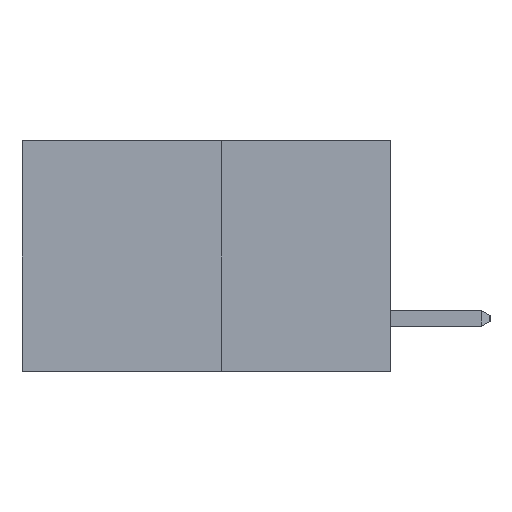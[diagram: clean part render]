
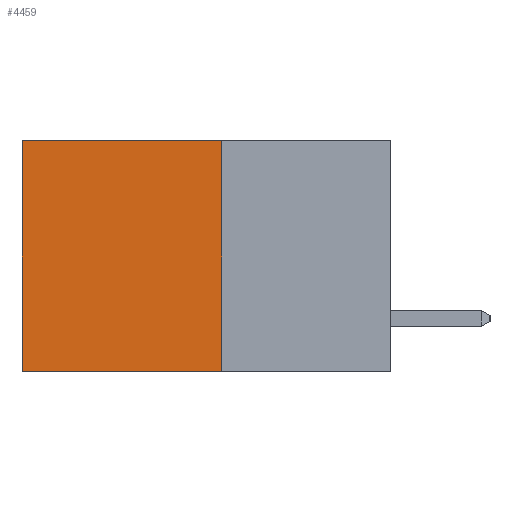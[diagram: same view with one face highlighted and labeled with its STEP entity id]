
A CAD part, left-side view. The second image highlights one B-rep face of the part: STEP entity #4459.
In plain terms, the highlighted planar face has unit normal (-1, 0, 0).
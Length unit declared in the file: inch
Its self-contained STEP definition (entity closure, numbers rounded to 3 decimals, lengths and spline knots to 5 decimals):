
#41 = FACE_OUTER_BOUND ( 'NONE', #4753, .T. ) ;
#660 = VECTOR ( 'NONE', #13528, 39.37008 ) ;
#2257 = CARTESIAN_POINT ( 'NONE',  ( 0.277, 0.27, 0. ) ) ;
#2770 = CARTESIAN_POINT ( 'NONE',  ( 0.277, 0.59, -0.37 ) ) ;
#2908 = CARTESIAN_POINT ( 'NONE',  ( 0.277, 0.27, 0. ) ) ;
#2916 = VERTEX_POINT ( 'NONE', #6749 ) ;
#3190 = LINE ( 'NONE', #10766, #14870 ) ;
#3522 = VERTEX_POINT ( 'NONE', #2257 ) ;
#3648 = EDGE_CURVE ( 'NONE', #2916, #9397, #7498, .T. ) ;
#4135 = DIRECTION ( 'NONE',  ( 0., 1., 0. ) ) ;
#4351 = DIRECTION ( 'NONE',  ( 0., 0., -1. ) ) ;
#4369 = DIRECTION ( 'NONE',  ( 1., 0., 0. ) ) ;
#4402 = CARTESIAN_POINT ( 'NONE',  ( 0.277, 0.27, -0.37 ) ) ;
#4459 = ADVANCED_FACE ( 'NONE', ( #41 ), #4654, .F. ) ;
#4654 = PLANE ( 'NONE',  #10296 ) ;
#4753 = EDGE_LOOP ( 'NONE', ( #5326, #5476, #5497, #5720 ) ) ;
#5326 = ORIENTED_EDGE ( 'NONE', *, *, #3648, .T. ) ;
#5476 = ORIENTED_EDGE ( 'NONE', *, *, #12457, .F. ) ;
#5497 = ORIENTED_EDGE ( 'NONE', *, *, #13616, .F. ) ;
#5720 = ORIENTED_EDGE ( 'NONE', *, *, #10115, .T. ) ;
#5869 = VECTOR ( 'NONE', #4135, 39.37008 ) ;
#6749 = CARTESIAN_POINT ( 'NONE',  ( 0.277, 0.59, 0. ) ) ;
#6946 = VECTOR ( 'NONE', #14303, 39.37008 ) ;
#7498 = LINE ( 'NONE', #13860, #660 ) ;
#8808 = CARTESIAN_POINT ( 'NONE',  ( 0.277, 0.27, -0.37 ) ) ;
#8969 = VERTEX_POINT ( 'NONE', #9063 ) ;
#9063 = CARTESIAN_POINT ( 'NONE',  ( 0.277, 0.27, -0.37 ) ) ;
#9264 = LINE ( 'NONE', #2908, #5869 ) ;
#9397 = VERTEX_POINT ( 'NONE', #2770 ) ;
#10115 = EDGE_CURVE ( 'NONE', #3522, #2916, #9264, .T. ) ;
#10296 = AXIS2_PLACEMENT_3D ( 'NONE', #4402, #4369, #4351 ) ;
#10766 = CARTESIAN_POINT ( 'NONE',  ( 0.277, 0.27, -0.37 ) ) ;
#12457 = EDGE_CURVE ( 'NONE', #8969, #9397, #13299, .T. ) ;
#13299 = LINE ( 'NONE', #8808, #6946 ) ;
#13528 = DIRECTION ( 'NONE',  ( 0., 0., -1. ) ) ;
#13616 = EDGE_CURVE ( 'NONE', #3522, #8969, #3190, .T. ) ;
#13860 = CARTESIAN_POINT ( 'NONE',  ( 0.277, 0.59, -0.37 ) ) ;
#14068 = DIRECTION ( 'NONE',  ( 0., 0., -1. ) ) ;
#14303 = DIRECTION ( 'NONE',  ( 0., 1., 0. ) ) ;
#14870 = VECTOR ( 'NONE', #14068, 39.37008 ) ;
